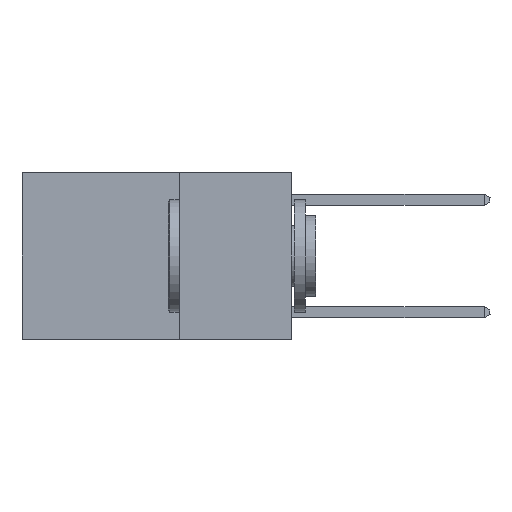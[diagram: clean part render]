
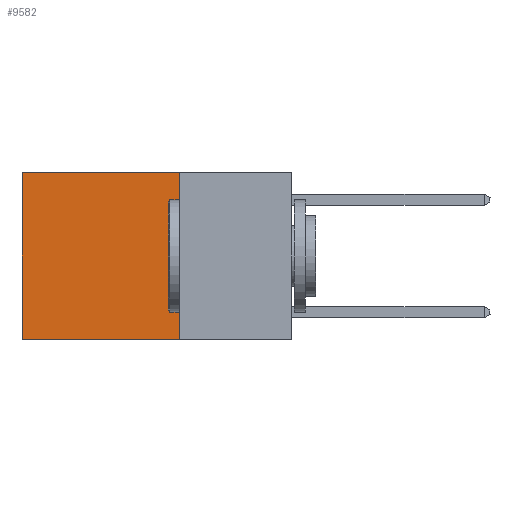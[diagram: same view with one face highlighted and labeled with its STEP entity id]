
A CAD part, left-side view. The second image highlights one B-rep face of the part: STEP entity #9582.
In plain terms, the highlighted planar face has unit normal (-1, 0, 0).
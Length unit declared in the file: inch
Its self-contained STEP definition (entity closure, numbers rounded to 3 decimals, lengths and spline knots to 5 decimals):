
#25 = DIRECTION ( 'NONE',  ( 0., 0., -1. ) ) ;
#1850 = PLANE ( 'NONE',  #16081 ) ;
#1920 = EDGE_LOOP ( 'NONE', ( #30387, #15983, #26126, #20464 ) ) ;
#2579 = VERTEX_POINT ( 'NONE', #29926 ) ;
#5670 = CARTESIAN_POINT ( 'NONE',  ( 0.2625, 0.6, 0. ) ) ;
#6346 = CARTESIAN_POINT ( 'NONE',  ( 0.2625, 0.25, -0.37 ) ) ;
#6468 = VERTEX_POINT ( 'NONE', #23180 ) ;
#7075 = CARTESIAN_POINT ( 'NONE',  ( 0.2625, 0.6, 0. ) ) ;
#7229 = CARTESIAN_POINT ( 'NONE',  ( 0.2625, 0.25, 0. ) ) ;
#8790 = EDGE_CURVE ( 'NONE', #10966, #6468, #25850, .T. ) ;
#9582 = ADVANCED_FACE ( 'NONE', ( #19774 ), #1850, .F. ) ;
#10966 = VERTEX_POINT ( 'NONE', #7075 ) ;
#11085 = CARTESIAN_POINT ( 'NONE',  ( 0.2625, 0.25, 0. ) ) ;
#13670 = LINE ( 'NONE', #6346, #21963 ) ;
#15323 = VECTOR ( 'NONE', #19549, 39.37008 ) ;
#15983 = ORIENTED_EDGE ( 'NONE', *, *, #27829, .F. ) ;
#16013 = VECTOR ( 'NONE', #30396, 39.37008 ) ;
#16081 = AXIS2_PLACEMENT_3D ( 'NONE', #7229, #24647, #25 ) ;
#17846 = VECTOR ( 'NONE', #21516, 39.37008 ) ;
#18592 = LINE ( 'NONE', #11085, #17846 ) ;
#19549 = DIRECTION ( 'NONE',  ( 0., 1., 0. ) ) ;
#19774 = FACE_OUTER_BOUND ( 'NONE', #1920, .T. ) ;
#20464 = ORIENTED_EDGE ( 'NONE', *, *, #30448, .T. ) ;
#21184 = LINE ( 'NONE', #27355, #15323 ) ;
#21516 = DIRECTION ( 'NONE',  ( 0., 0., -1. ) ) ;
#21963 = VECTOR ( 'NONE', #26218, 39.37008 ) ;
#23180 = CARTESIAN_POINT ( 'NONE',  ( 0.2625, 0.6, -0.37 ) ) ;
#24533 = EDGE_CURVE ( 'NONE', #25863, #2579, #18592, .T. ) ;
#24647 = DIRECTION ( 'NONE',  ( 1., 0., 0. ) ) ;
#25850 = LINE ( 'NONE', #5670, #16013 ) ;
#25863 = VERTEX_POINT ( 'NONE', #28993 ) ;
#26126 = ORIENTED_EDGE ( 'NONE', *, *, #24533, .F. ) ;
#26218 = DIRECTION ( 'NONE',  ( 0., 1., 0. ) ) ;
#27355 = CARTESIAN_POINT ( 'NONE',  ( 0.2625, 0.25, 0. ) ) ;
#27829 = EDGE_CURVE ( 'NONE', #2579, #6468, #13670, .T. ) ;
#28993 = CARTESIAN_POINT ( 'NONE',  ( 0.2625, 0.25, 0. ) ) ;
#29926 = CARTESIAN_POINT ( 'NONE',  ( 0.2625, 0.25, -0.37 ) ) ;
#30387 = ORIENTED_EDGE ( 'NONE', *, *, #8790, .T. ) ;
#30396 = DIRECTION ( 'NONE',  ( 0., 0., -1. ) ) ;
#30448 = EDGE_CURVE ( 'NONE', #25863, #10966, #21184, .T. ) ;
